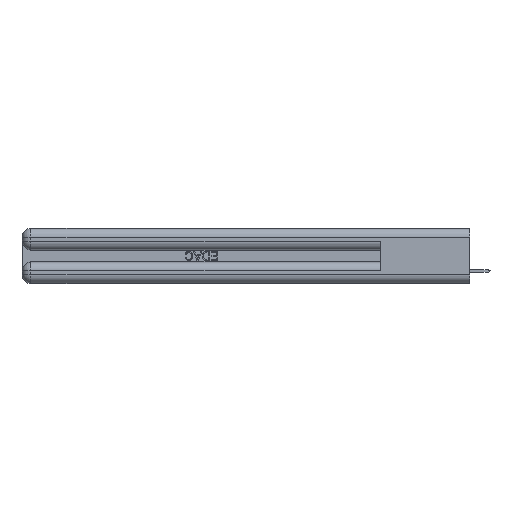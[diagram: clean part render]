
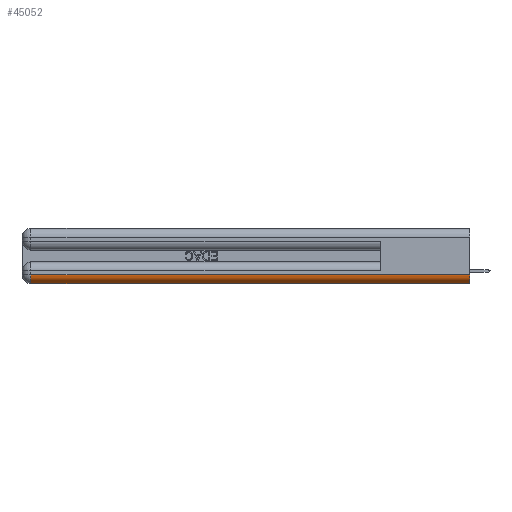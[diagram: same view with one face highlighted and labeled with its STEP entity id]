
A CAD part, left-side view. The second image highlights one B-rep face of the part: STEP entity #45052.
In plain terms, the highlighted cylindrical face has radius 1.524 mm (diameter 3.048 mm), a partial arc.
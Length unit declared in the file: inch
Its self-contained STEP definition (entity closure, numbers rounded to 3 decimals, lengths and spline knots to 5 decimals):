
#40 = CARTESIAN_POINT ( 'NONE',  ( 0., 0., 0.06 ) ) ;
#916 = VERTEX_POINT ( 'NONE', #41440 ) ;
#1323 = CARTESIAN_POINT ( 'NONE',  ( 0.06, 3., 0. ) ) ;
#5075 = VECTOR ( 'NONE', #34784, 39.37008 ) ;
#5865 = CARTESIAN_POINT ( 'NONE',  ( 0.06, 0., 0.06 ) ) ;
#6181 = CARTESIAN_POINT ( 'NONE',  ( 0., 2.94, 0.06 ) ) ;
#7324 = ORIENTED_EDGE ( 'NONE', *, *, #42077, .F. ) ;
#8696 = CYLINDRICAL_SURFACE ( 'NONE', #13802, 0.06 ) ;
#9992 = FACE_OUTER_BOUND ( 'NONE', #38687, .T. ) ;
#10350 = CARTESIAN_POINT ( 'NONE',  ( 0., 0., 0.06 ) ) ;
#13654 = LINE ( 'NONE', #10350, #5075 ) ;
#13802 = AXIS2_PLACEMENT_3D ( 'NONE', #5865, #51964, #38078 ) ;
#14560 = CARTESIAN_POINT ( 'NONE',  ( 0.06, 0., 0. ) ) ;
#15803 = EDGE_CURVE ( 'NONE', #916, #29363, #20829, .T. ) ;
#17103 = DIRECTION ( 'NONE',  ( 0., -1., 0. ) ) ;
#18054 = DIRECTION ( 'NONE',  ( 0., 1., 0. ) ) ;
#19051 = AXIS2_PLACEMENT_3D ( 'NONE', #19621, #28147, #41006 ) ;
#19621 = CARTESIAN_POINT ( 'NONE',  ( 0.06, 2.94, 0.06 ) ) ;
#20829 = CIRCLE ( 'NONE', #19051, 0.06 ) ;
#21950 = VERTEX_POINT ( 'NONE', #40 ) ;
#23842 = DIRECTION ( 'NONE',  ( 0., 0., 1. ) ) ;
#25053 = VECTOR ( 'NONE', #18054, 39.37008 ) ;
#28147 = DIRECTION ( 'NONE',  ( 0., 1., 0. ) ) ;
#29363 = VERTEX_POINT ( 'NONE', #6181 ) ;
#31891 = EDGE_CURVE ( 'NONE', #29363, #21950, #13654, .T. ) ;
#32960 = ORIENTED_EDGE ( 'NONE', *, *, #15803, .F. ) ;
#33559 = ORIENTED_EDGE ( 'NONE', *, *, #31891, .F. ) ;
#33584 = VERTEX_POINT ( 'NONE', #14560 ) ;
#34160 = EDGE_CURVE ( 'NONE', #21950, #33584, #37754, .T. ) ;
#34784 = DIRECTION ( 'NONE',  ( 0., -1., 0. ) ) ;
#35494 = ORIENTED_EDGE ( 'NONE', *, *, #34160, .F. ) ;
#37754 = CIRCLE ( 'NONE', #47390, 0.06 ) ;
#38078 = DIRECTION ( 'NONE',  ( 0., 0., 1. ) ) ;
#38687 = EDGE_LOOP ( 'NONE', ( #35494, #33559, #32960, #7324 ) ) ;
#41006 = DIRECTION ( 'NONE',  ( 0., 0., 1. ) ) ;
#41440 = CARTESIAN_POINT ( 'NONE',  ( 0.06, 2.94, 0. ) ) ;
#42077 = EDGE_CURVE ( 'NONE', #33584, #916, #47144, .T. ) ;
#45052 = ADVANCED_FACE ( 'NONE', ( #9992 ), #8696, .T. ) ;
#47144 = LINE ( 'NONE', #1323, #25053 ) ;
#47390 = AXIS2_PLACEMENT_3D ( 'NONE', #50338, #17103, #23842 ) ;
#50338 = CARTESIAN_POINT ( 'NONE',  ( 0.06, 0., 0.06 ) ) ;
#51964 = DIRECTION ( 'NONE',  ( 0., 1., 0. ) ) ;
